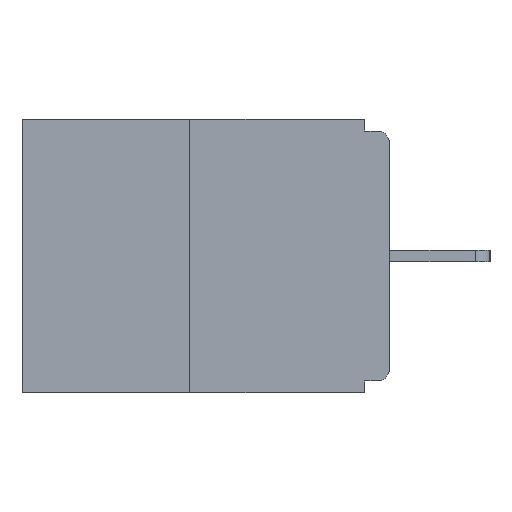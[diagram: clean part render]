
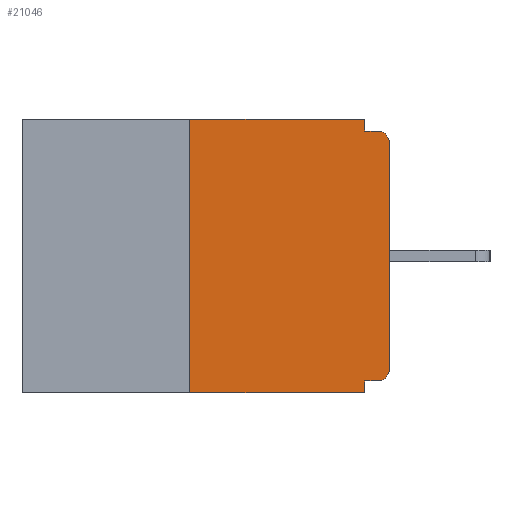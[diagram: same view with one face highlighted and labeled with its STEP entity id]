
A CAD part, left-side view. The second image highlights one B-rep face of the part: STEP entity #21046.
In plain terms, the highlighted planar face has unit normal (-1, 0, 0).
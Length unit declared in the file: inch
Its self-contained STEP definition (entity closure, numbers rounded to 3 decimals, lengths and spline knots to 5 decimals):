
#305 = CIRCLE ( 'NONE', #5055, 0.015 ) ;
#820 = CARTESIAN_POINT ( 'NONE',  ( 0., 0., -0.015 ) ) ;
#1461 = CARTESIAN_POINT ( 'NONE',  ( 0., 0., -0.03 ) ) ;
#1477 = EDGE_CURVE ( 'NONE', #13947, #14161, #13494, .T. ) ;
#1801 = DIRECTION ( 'NONE',  ( 0., -1., 0. ) ) ;
#1852 = CARTESIAN_POINT ( 'NONE',  ( 0., 0.031, -0.343 ) ) ;
#1866 = DIRECTION ( 'NONE',  ( 0., -1., 0. ) ) ;
#1870 = CARTESIAN_POINT ( 'NONE',  ( 0., 0.46, 0. ) ) ;
#2009 = PLANE ( 'NONE',  #8471 ) ;
#2095 = ORIENTED_EDGE ( 'NONE', *, *, #14500, .T. ) ;
#2120 = CIRCLE ( 'NONE', #25435, 0.015 ) ;
#2966 = CARTESIAN_POINT ( 'NONE',  ( 0., 0.25, -0.343 ) ) ;
#3387 = ORIENTED_EDGE ( 'NONE', *, *, #1477, .T. ) ;
#4605 = VECTOR ( 'NONE', #16369, 39.37008 ) ;
#4678 = ORIENTED_EDGE ( 'NONE', *, *, #4755, .F. ) ;
#4755 = EDGE_CURVE ( 'NONE', #12152, #18688, #18695, .T. ) ;
#5055 = AXIS2_PLACEMENT_3D ( 'NONE', #21446, #9391, #23412 ) ;
#6216 = CARTESIAN_POINT ( 'NONE',  ( 0., 0.031, -0.343 ) ) ;
#6385 = CARTESIAN_POINT ( 'NONE',  ( 0., 0.031, 0. ) ) ;
#6400 = CARTESIAN_POINT ( 'NONE',  ( 0., 0.015, -0.015 ) ) ;
#6685 = ORIENTED_EDGE ( 'NONE', *, *, #10080, .F. ) ;
#6789 = CARTESIAN_POINT ( 'NONE',  ( 0., 0.46, -0.343 ) ) ;
#6934 = LINE ( 'NONE', #1870, #23003 ) ;
#7838 = VECTOR ( 'NONE', #8850, 39.37008 ) ;
#7952 = VECTOR ( 'NONE', #1801, 39.37008 ) ;
#8095 = VECTOR ( 'NONE', #13859, 39.37008 ) ;
#8259 = DIRECTION ( 'NONE',  ( 0., 0., -1. ) ) ;
#8471 = AXIS2_PLACEMENT_3D ( 'NONE', #26220, #20362, #8259 ) ;
#8510 = CARTESIAN_POINT ( 'NONE',  ( 0., 0.015, -0.03 ) ) ;
#8833 = DIRECTION ( 'NONE',  ( 0., 0., 1. ) ) ;
#8850 = DIRECTION ( 'NONE',  ( 0., -1., 0. ) ) ;
#9391 = DIRECTION ( 'NONE',  ( -1., 0., 0. ) ) ;
#9586 = VERTEX_POINT ( 'NONE', #13046 ) ;
#9711 = DIRECTION ( 'NONE',  ( 0., 0., -1. ) ) ;
#9924 = LINE ( 'NONE', #22895, #20005 ) ;
#10080 = EDGE_CURVE ( 'NONE', #9586, #15952, #6934, .T. ) ;
#10449 = EDGE_CURVE ( 'NONE', #15952, #12152, #14862, .T. ) ;
#10573 = DIRECTION ( 'NONE',  ( 0., 0., -1. ) ) ;
#10690 = VERTEX_POINT ( 'NONE', #18508 ) ;
#10754 = CARTESIAN_POINT ( 'NONE',  ( 0., 0., -0.328 ) ) ;
#11116 = CARTESIAN_POINT ( 'NONE',  ( 0., 0., -0.313 ) ) ;
#12152 = VERTEX_POINT ( 'NONE', #19221 ) ;
#12501 = VERTEX_POINT ( 'NONE', #24743 ) ;
#13014 = ORIENTED_EDGE ( 'NONE', *, *, #13158, .F. ) ;
#13046 = CARTESIAN_POINT ( 'NONE',  ( 0., 0.25, 0. ) ) ;
#13158 = EDGE_CURVE ( 'NONE', #12501, #15849, #14221, .T. ) ;
#13494 = LINE ( 'NONE', #14655, #8095 ) ;
#13859 = DIRECTION ( 'NONE',  ( 0., 0., 1. ) ) ;
#13947 = VERTEX_POINT ( 'NONE', #11116 ) ;
#14161 = VERTEX_POINT ( 'NONE', #1461 ) ;
#14221 = LINE ( 'NONE', #6216, #4605 ) ;
#14243 = VECTOR ( 'NONE', #9711, 39.37008 ) ;
#14343 = EDGE_LOOP ( 'NONE', ( #6685, #17104, #2095, #13014, #23642, #24260, #3387, #25504, #4678, #21523 ) ) ;
#14500 = EDGE_CURVE ( 'NONE', #26126, #15849, #23853, .T. ) ;
#14655 = CARTESIAN_POINT ( 'NONE',  ( 0., 0., 0. ) ) ;
#14808 = DIRECTION ( 'NONE',  ( 0., 1., 0. ) ) ;
#14862 = LINE ( 'NONE', #19760, #14243 ) ;
#14962 = FACE_OUTER_BOUND ( 'NONE', #14343, .T. ) ;
#15714 = EDGE_CURVE ( 'NONE', #10690, #12501, #25643, .T. ) ;
#15849 = VERTEX_POINT ( 'NONE', #1852 ) ;
#15952 = VERTEX_POINT ( 'NONE', #6385 ) ;
#16369 = DIRECTION ( 'NONE',  ( 0., 0., -1. ) ) ;
#17104 = ORIENTED_EDGE ( 'NONE', *, *, #17203, .F. ) ;
#17203 = EDGE_CURVE ( 'NONE', #26126, #9586, #9924, .T. ) ;
#18508 = CARTESIAN_POINT ( 'NONE',  ( 0., 0.015, -0.328 ) ) ;
#18688 = VERTEX_POINT ( 'NONE', #6400 ) ;
#18695 = LINE ( 'NONE', #820, #7952 ) ;
#19221 = CARTESIAN_POINT ( 'NONE',  ( 0., 0.031, -0.015 ) ) ;
#19760 = CARTESIAN_POINT ( 'NONE',  ( 0., 0.031, 0. ) ) ;
#20005 = VECTOR ( 'NONE', #8833, 39.37008 ) ;
#20362 = DIRECTION ( 'NONE',  ( 1., 0., 0. ) ) ;
#20405 = VECTOR ( 'NONE', #14808, 39.37008 ) ;
#21046 = ADVANCED_FACE ( 'NONE', ( #14962 ), #2009, .F. ) ;
#21446 = CARTESIAN_POINT ( 'NONE',  ( 0., 0.015, -0.313 ) ) ;
#21523 = ORIENTED_EDGE ( 'NONE', *, *, #10449, .F. ) ;
#21594 = EDGE_CURVE ( 'NONE', #14161, #18688, #2120, .T. ) ;
#22588 = DIRECTION ( 'NONE',  ( -1., 0., 0. ) ) ;
#22895 = CARTESIAN_POINT ( 'NONE',  ( 0., 0.25, 0. ) ) ;
#23003 = VECTOR ( 'NONE', #1866, 39.37008 ) ;
#23412 = DIRECTION ( 'NONE',  ( 0., 0., -1. ) ) ;
#23642 = ORIENTED_EDGE ( 'NONE', *, *, #15714, .F. ) ;
#23853 = LINE ( 'NONE', #6789, #7838 ) ;
#24200 = EDGE_CURVE ( 'NONE', #10690, #13947, #305, .T. ) ;
#24260 = ORIENTED_EDGE ( 'NONE', *, *, #24200, .T. ) ;
#24743 = CARTESIAN_POINT ( 'NONE',  ( 0., 0.031, -0.328 ) ) ;
#25435 = AXIS2_PLACEMENT_3D ( 'NONE', #8510, #22588, #10573 ) ;
#25504 = ORIENTED_EDGE ( 'NONE', *, *, #21594, .T. ) ;
#25643 = LINE ( 'NONE', #10754, #20405 ) ;
#26126 = VERTEX_POINT ( 'NONE', #2966 ) ;
#26220 = CARTESIAN_POINT ( 'NONE',  ( 0., 0.46, 0. ) ) ;
